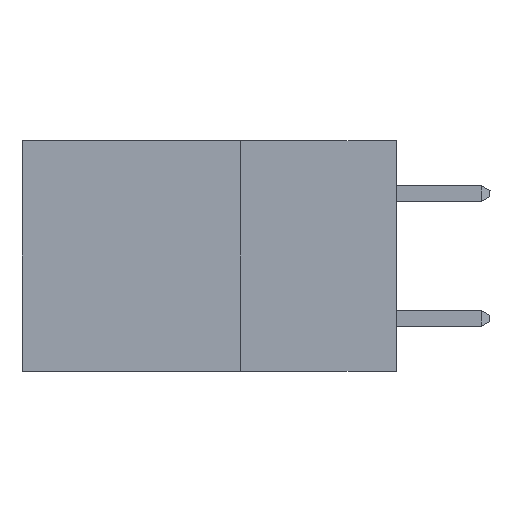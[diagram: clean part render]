
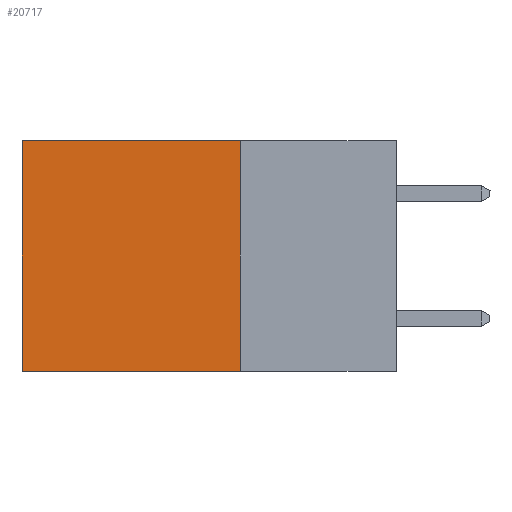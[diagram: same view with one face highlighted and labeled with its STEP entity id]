
A CAD part, left-side view. The second image highlights one B-rep face of the part: STEP entity #20717.
In plain terms, the highlighted planar face has unit normal (-1, 0, 0).
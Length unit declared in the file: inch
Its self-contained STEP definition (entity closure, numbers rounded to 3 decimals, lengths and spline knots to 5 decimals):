
#1135 = ORIENTED_EDGE ( 'NONE', *, *, #19989, .F. ) ;
#1911 = CARTESIAN_POINT ( 'NONE',  ( 0.298, 0.25, -0.37 ) ) ;
#2525 = ORIENTED_EDGE ( 'NONE', *, *, #29074, .T. ) ;
#3067 = LINE ( 'NONE', #24464, #15198 ) ;
#4130 = VERTEX_POINT ( 'NONE', #28765 ) ;
#5532 = EDGE_LOOP ( 'NONE', ( #2525, #1135, #11730, #29517 ) ) ;
#7594 = DIRECTION ( 'NONE',  ( 1., 0., 0. ) ) ;
#9952 = CARTESIAN_POINT ( 'NONE',  ( 0.298, 0.25, 0. ) ) ;
#10918 = DIRECTION ( 'NONE',  ( 0., 0., -1. ) ) ;
#11730 = ORIENTED_EDGE ( 'NONE', *, *, #20286, .F. ) ;
#13029 = AXIS2_PLACEMENT_3D ( 'NONE', #9952, #7594, #24659 ) ;
#13927 = CARTESIAN_POINT ( 'NONE',  ( 0.298, 0.6, 0. ) ) ;
#14204 = LINE ( 'NONE', #18245, #20704 ) ;
#15198 = VECTOR ( 'NONE', #24360, 39.37008 ) ;
#16981 = FACE_OUTER_BOUND ( 'NONE', #5532, .T. ) ;
#18245 = CARTESIAN_POINT ( 'NONE',  ( 0.298, 0.6, 0. ) ) ;
#18291 = CARTESIAN_POINT ( 'NONE',  ( 0.298, 0.25, 0. ) ) ;
#18508 = VERTEX_POINT ( 'NONE', #1911 ) ;
#19989 = EDGE_CURVE ( 'NONE', #18508, #22350, #30948, .T. ) ;
#20286 = EDGE_CURVE ( 'NONE', #4130, #18508, #29817, .T. ) ;
#20704 = VECTOR ( 'NONE', #27944, 39.37008 ) ;
#20717 = ADVANCED_FACE ( 'NONE', ( #16981 ), #22233, .F. ) ;
#20869 = CARTESIAN_POINT ( 'NONE',  ( 0.298, 0.6, -0.37 ) ) ;
#22233 = PLANE ( 'NONE',  #13029 ) ;
#22350 = VERTEX_POINT ( 'NONE', #20869 ) ;
#24178 = CARTESIAN_POINT ( 'NONE',  ( 0.298, 0.25, -0.37 ) ) ;
#24296 = VECTOR ( 'NONE', #10918, 39.37008 ) ;
#24360 = DIRECTION ( 'NONE',  ( 0., 1., 0. ) ) ;
#24421 = VERTEX_POINT ( 'NONE', #13927 ) ;
#24464 = CARTESIAN_POINT ( 'NONE',  ( 0.298, 0.25, 0. ) ) ;
#24659 = DIRECTION ( 'NONE',  ( 0., 0., -1. ) ) ;
#24676 = VECTOR ( 'NONE', #28918, 39.37008 ) ;
#25164 = EDGE_CURVE ( 'NONE', #4130, #24421, #3067, .T. ) ;
#27944 = DIRECTION ( 'NONE',  ( 0., 0., -1. ) ) ;
#28765 = CARTESIAN_POINT ( 'NONE',  ( 0.298, 0.25, 0. ) ) ;
#28918 = DIRECTION ( 'NONE',  ( 0., 1., 0. ) ) ;
#29074 = EDGE_CURVE ( 'NONE', #24421, #22350, #14204, .T. ) ;
#29517 = ORIENTED_EDGE ( 'NONE', *, *, #25164, .T. ) ;
#29817 = LINE ( 'NONE', #18291, #24296 ) ;
#30948 = LINE ( 'NONE', #24178, #24676 ) ;
